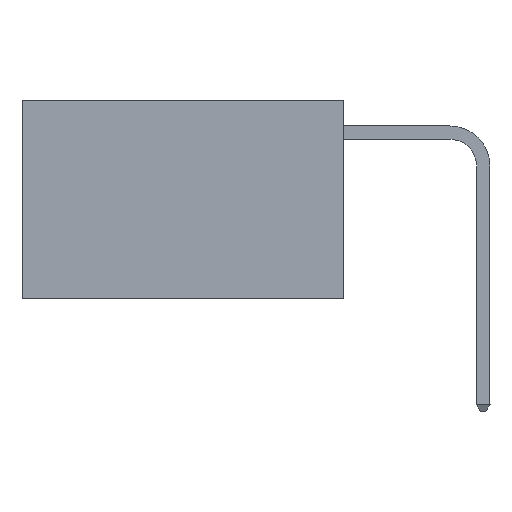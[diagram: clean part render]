
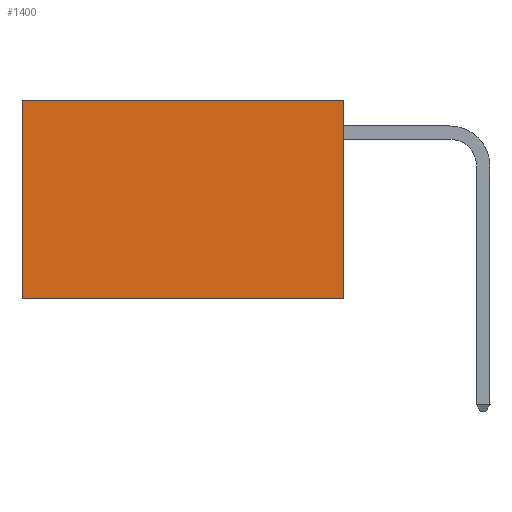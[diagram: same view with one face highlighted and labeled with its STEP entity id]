
A CAD part, left-side view. The second image highlights one B-rep face of the part: STEP entity #1400.
In plain terms, the highlighted planar face has unit normal (-1, 0, 0).
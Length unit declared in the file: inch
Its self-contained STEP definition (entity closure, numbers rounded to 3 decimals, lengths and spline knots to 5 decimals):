
#23 = CARTESIAN_POINT ( 'NONE',  ( 0.2625, 0., 0. ) ) ;
#196 = CARTESIAN_POINT ( 'NONE',  ( 0.2625, 0., 0. ) ) ;
#562 = ORIENTED_EDGE ( 'NONE', *, *, #7077, .T. ) ;
#935 = ORIENTED_EDGE ( 'NONE', *, *, #6503, .F. ) ;
#1400 = ADVANCED_FACE ( 'NONE', ( #4385 ), #2613, .F. ) ;
#1402 = CARTESIAN_POINT ( 'NONE',  ( 0.2625, 0., 0. ) ) ;
#1445 = ORIENTED_EDGE ( 'NONE', *, *, #9397, .F. ) ;
#1521 = ORIENTED_EDGE ( 'NONE', *, *, #5831, .T. ) ;
#1875 = DIRECTION ( 'NONE',  ( 0., 1., 0. ) ) ;
#2073 = CARTESIAN_POINT ( 'NONE',  ( 0.2625, 0.6, 0. ) ) ;
#2542 = VECTOR ( 'NONE', #3353, 39.37008 ) ;
#2613 = PLANE ( 'NONE',  #3682 ) ;
#3244 = VECTOR ( 'NONE', #6763, 39.37008 ) ;
#3353 = DIRECTION ( 'NONE',  ( 0., 0., -1. ) ) ;
#3682 = AXIS2_PLACEMENT_3D ( 'NONE', #23, #9585, #5262 ) ;
#4042 = LINE ( 'NONE', #5927, #3244 ) ;
#4048 = LINE ( 'NONE', #1402, #2542 ) ;
#4239 = CARTESIAN_POINT ( 'NONE',  ( 0.2625, 0.6, 0. ) ) ;
#4385 = FACE_OUTER_BOUND ( 'NONE', #10355, .T. ) ;
#4388 = LINE ( 'NONE', #196, #7212 ) ;
#4582 = CARTESIAN_POINT ( 'NONE',  ( 0.2625, 0., -0.37 ) ) ;
#5262 = DIRECTION ( 'NONE',  ( 0., 0., -1. ) ) ;
#5810 = CARTESIAN_POINT ( 'NONE',  ( 0.2625, 0., 0. ) ) ;
#5831 = EDGE_CURVE ( 'NONE', #9927, #6726, #4388, .T. ) ;
#5927 = CARTESIAN_POINT ( 'NONE',  ( 0.2625, 0., -0.37 ) ) ;
#6159 = VERTEX_POINT ( 'NONE', #6723 ) ;
#6503 = EDGE_CURVE ( 'NONE', #6761, #6159, #4042, .T. ) ;
#6723 = CARTESIAN_POINT ( 'NONE',  ( 0.2625, 0.6, -0.37 ) ) ;
#6726 = VERTEX_POINT ( 'NONE', #2073 ) ;
#6761 = VERTEX_POINT ( 'NONE', #4582 ) ;
#6763 = DIRECTION ( 'NONE',  ( 0., 1., 0. ) ) ;
#6797 = LINE ( 'NONE', #4239, #7974 ) ;
#7077 = EDGE_CURVE ( 'NONE', #6726, #6159, #6797, .T. ) ;
#7212 = VECTOR ( 'NONE', #1875, 39.37008 ) ;
#7974 = VECTOR ( 'NONE', #10300, 39.37008 ) ;
#9397 = EDGE_CURVE ( 'NONE', #9927, #6761, #4048, .T. ) ;
#9585 = DIRECTION ( 'NONE',  ( 1., 0., 0. ) ) ;
#9927 = VERTEX_POINT ( 'NONE', #5810 ) ;
#10300 = DIRECTION ( 'NONE',  ( 0., 0., -1. ) ) ;
#10355 = EDGE_LOOP ( 'NONE', ( #562, #935, #1445, #1521 ) ) ;
